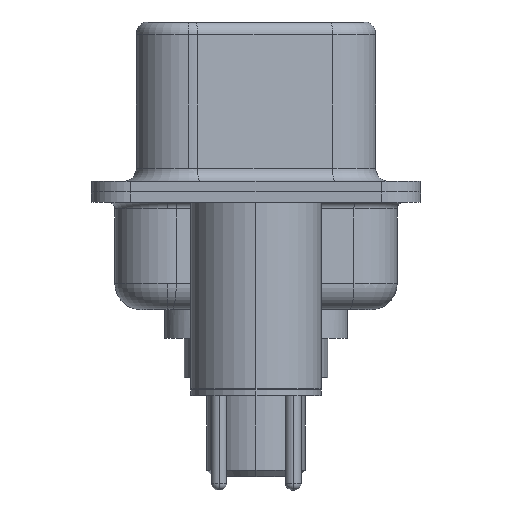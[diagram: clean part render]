
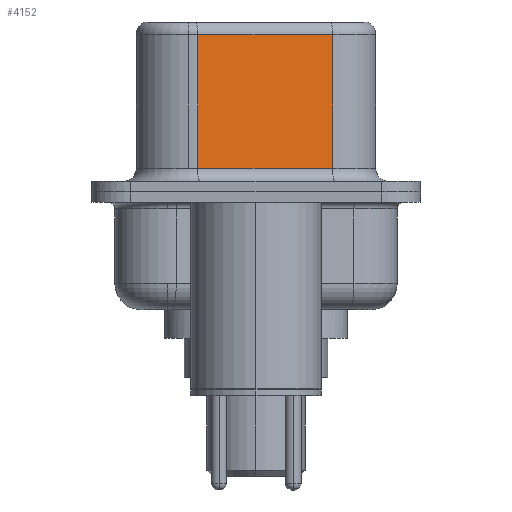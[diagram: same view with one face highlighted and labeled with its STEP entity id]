
A CAD part, left-side view. The second image highlights one B-rep face of the part: STEP entity #4152.
In plain terms, the highlighted planar face has unit normal (-0.985, -0.174, 0).
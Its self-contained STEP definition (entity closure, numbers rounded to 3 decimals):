
#186 = EDGE_CURVE ( 'NONE', #16392, #20931, #4333, .T. ) ;
#610 = CARTESIAN_POINT ( 'NONE',  ( 3.655, 2.233, 6.02 ) ) ;
#971 = ORIENTED_EDGE ( 'NONE', *, *, #186, .F. ) ;
#1812 = DIRECTION ( 'NONE',  ( -0.174, 0.985, 0. ) ) ;
#2581 = CARTESIAN_POINT ( 'NONE',  ( 4.565, -2.927, 6.52 ) ) ;
#2831 = VECTOR ( 'NONE', #1812, 1000. ) ;
#3067 = LINE ( 'NONE', #3348, #19563 ) ;
#3348 = CARTESIAN_POINT ( 'NONE',  ( 3.655, 2.233, 6.52 ) ) ;
#3526 = ORIENTED_EDGE ( 'NONE', *, *, #4460, .T. ) ;
#3884 = DIRECTION ( 'NONE',  ( 0., 0., -1. ) ) ;
#4152 = ADVANCED_FACE ( 'NONE', ( #11519 ), #19231, .F. ) ;
#4232 = LINE ( 'NONE', #16896, #21243 ) ;
#4333 = LINE ( 'NONE', #2581, #21349 ) ;
#4460 = EDGE_CURVE ( 'NONE', #8067, #5247, #3067, .T. ) ;
#4597 = ORIENTED_EDGE ( 'NONE', *, *, #9832, .T. ) ;
#5247 = VERTEX_POINT ( 'NONE', #6688 ) ;
#6688 = CARTESIAN_POINT ( 'NONE',  ( 3.655, 2.233, 0.9 ) ) ;
#7669 = CARTESIAN_POINT ( 'NONE',  ( 4.565, -2.927, 6.02 ) ) ;
#8067 = VERTEX_POINT ( 'NONE', #610 ) ;
#9248 = EDGE_LOOP ( 'NONE', ( #971, #4597, #3526, #19601 ) ) ;
#9618 = DIRECTION ( 'NONE',  ( -0.174, 0.985, 0. ) ) ;
#9832 = EDGE_CURVE ( 'NONE', #16392, #8067, #11533, .T. ) ;
#10949 = CARTESIAN_POINT ( 'NONE',  ( 4.565, -2.927, 6.52 ) ) ;
#11519 = FACE_OUTER_BOUND ( 'NONE', #9248, .T. ) ;
#11533 = LINE ( 'NONE', #14959, #2831 ) ;
#12006 = DIRECTION ( 'NONE',  ( 0.174, -0.985, 0. ) ) ;
#14815 = CARTESIAN_POINT ( 'NONE',  ( 4.565, -2.927, 0.9 ) ) ;
#14831 = EDGE_CURVE ( 'NONE', #5247, #20931, #4232, .T. ) ;
#14959 = CARTESIAN_POINT ( 'NONE',  ( 4.565, -2.927, 6.02 ) ) ;
#15347 = DIRECTION ( 'NONE',  ( 0., 0., -1. ) ) ;
#16392 = VERTEX_POINT ( 'NONE', #7669 ) ;
#16499 = AXIS2_PLACEMENT_3D ( 'NONE', #10949, #20285, #9618 ) ;
#16896 = CARTESIAN_POINT ( 'NONE',  ( 4.565, -2.927, 0.9 ) ) ;
#19231 = PLANE ( 'NONE',  #16499 ) ;
#19563 = VECTOR ( 'NONE', #3884, 1000. ) ;
#19601 = ORIENTED_EDGE ( 'NONE', *, *, #14831, .T. ) ;
#20285 = DIRECTION ( 'NONE',  ( 0.985, 0.174, 0. ) ) ;
#20931 = VERTEX_POINT ( 'NONE', #14815 ) ;
#21243 = VECTOR ( 'NONE', #12006, 1000. ) ;
#21349 = VECTOR ( 'NONE', #15347, 1000. ) ;
